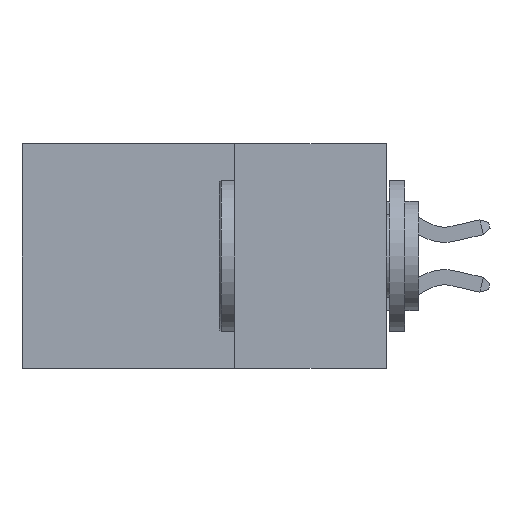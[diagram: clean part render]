
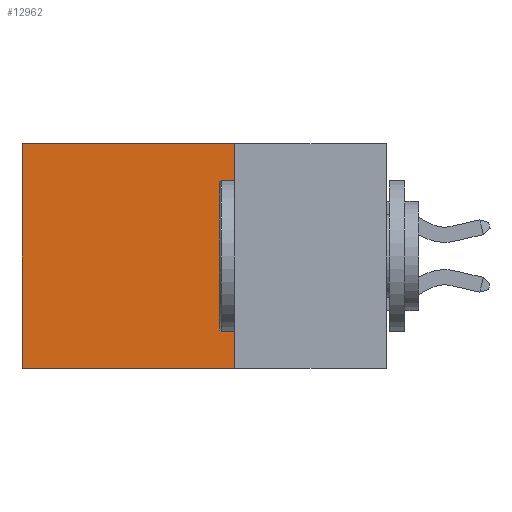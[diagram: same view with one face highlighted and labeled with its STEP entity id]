
A CAD part, left-side view. The second image highlights one B-rep face of the part: STEP entity #12962.
In plain terms, the highlighted planar face has unit normal (-1, 0, 0).
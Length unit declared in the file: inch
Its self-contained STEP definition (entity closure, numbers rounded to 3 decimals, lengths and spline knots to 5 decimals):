
#50 = VERTEX_POINT ( 'NONE', #8691 ) ;
#220 = DIRECTION ( 'NONE',  ( 1., 0., 0. ) ) ;
#737 = VERTEX_POINT ( 'NONE', #9344 ) ;
#1035 = CARTESIAN_POINT ( 'NONE',  ( 0.2615, 0.25, 0. ) ) ;
#1436 = CARTESIAN_POINT ( 'NONE',  ( 0.2615, 0.6, -0.37 ) ) ;
#1872 = EDGE_CURVE ( 'NONE', #13683, #15497, #14847, .T. ) ;
#2087 = CARTESIAN_POINT ( 'NONE',  ( 0.2615, 0.6, 0. ) ) ;
#2107 = EDGE_LOOP ( 'NONE', ( #11142, #12846, #8257, #14363 ) ) ;
#2364 = PLANE ( 'NONE',  #5581 ) ;
#3621 = VECTOR ( 'NONE', #11579, 39.37008 ) ;
#4303 = VECTOR ( 'NONE', #15011, 39.37008 ) ;
#4645 = VECTOR ( 'NONE', #7544, 39.37008 ) ;
#4716 = FACE_OUTER_BOUND ( 'NONE', #2107, .T. ) ;
#4944 = CARTESIAN_POINT ( 'NONE',  ( 0.2615, 0.25, -0.37 ) ) ;
#5581 = AXIS2_PLACEMENT_3D ( 'NONE', #14583, #220, #5890 ) ;
#5890 = DIRECTION ( 'NONE',  ( 0., 0., -1. ) ) ;
#6085 = EDGE_CURVE ( 'NONE', #15497, #50, #12144, .T. ) ;
#7544 = DIRECTION ( 'NONE',  ( 0., 0., -1. ) ) ;
#8257 = ORIENTED_EDGE ( 'NONE', *, *, #12911, .F. ) ;
#8691 = CARTESIAN_POINT ( 'NONE',  ( 0.2615, 0.6, -0.37 ) ) ;
#9344 = CARTESIAN_POINT ( 'NONE',  ( 0.2615, 0.25, -0.37 ) ) ;
#10785 = EDGE_CURVE ( 'NONE', #737, #50, #12382, .T. ) ;
#11019 = LINE ( 'NONE', #4944, #11119 ) ;
#11119 = VECTOR ( 'NONE', #14426, 39.37008 ) ;
#11142 = ORIENTED_EDGE ( 'NONE', *, *, #6085, .T. ) ;
#11579 = DIRECTION ( 'NONE',  ( 0., 1., 0. ) ) ;
#12144 = LINE ( 'NONE', #1436, #4645 ) ;
#12382 = LINE ( 'NONE', #14216, #3621 ) ;
#12846 = ORIENTED_EDGE ( 'NONE', *, *, #10785, .F. ) ;
#12911 = EDGE_CURVE ( 'NONE', #13683, #737, #11019, .T. ) ;
#12962 = ADVANCED_FACE ( 'NONE', ( #4716 ), #2364, .F. ) ;
#13666 = CARTESIAN_POINT ( 'NONE',  ( 0.2615, 0.25, 0. ) ) ;
#13683 = VERTEX_POINT ( 'NONE', #1035 ) ;
#14216 = CARTESIAN_POINT ( 'NONE',  ( 0.2615, 0.25, -0.37 ) ) ;
#14363 = ORIENTED_EDGE ( 'NONE', *, *, #1872, .T. ) ;
#14426 = DIRECTION ( 'NONE',  ( 0., 0., -1. ) ) ;
#14583 = CARTESIAN_POINT ( 'NONE',  ( 0.2615, 0.25, -0.37 ) ) ;
#14847 = LINE ( 'NONE', #13666, #4303 ) ;
#15011 = DIRECTION ( 'NONE',  ( 0., 1., 0. ) ) ;
#15497 = VERTEX_POINT ( 'NONE', #2087 ) ;
